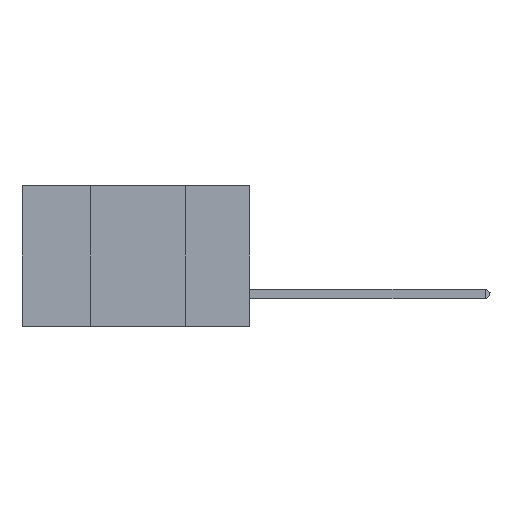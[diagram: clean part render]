
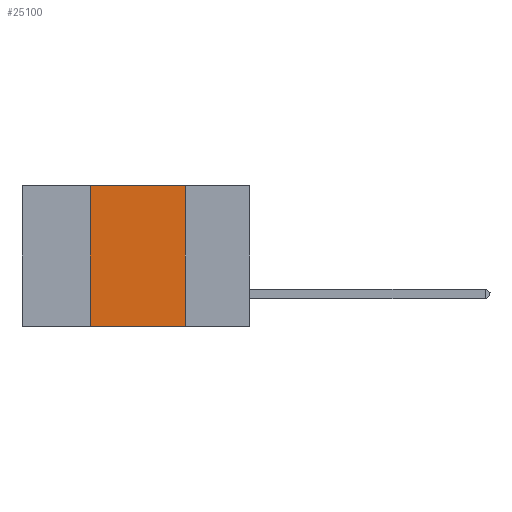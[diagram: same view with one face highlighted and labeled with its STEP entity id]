
A CAD part, left-side view. The second image highlights one B-rep face of the part: STEP entity #25100.
In plain terms, the highlighted planar face has unit normal (-1, 0, 0).
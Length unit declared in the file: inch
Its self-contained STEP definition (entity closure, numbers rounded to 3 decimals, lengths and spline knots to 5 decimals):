
#348 = LINE ( 'NONE', #39843, #4585 ) ;
#433 = VERTEX_POINT ( 'NONE', #11634 ) ;
#893 = DIRECTION ( 'NONE',  ( 0., -1., 0. ) ) ;
#2238 = CARTESIAN_POINT ( 'NONE',  ( 0., 0.42, 0. ) ) ;
#4585 = VECTOR ( 'NONE', #43239, 39.37008 ) ;
#5715 = VECTOR ( 'NONE', #893, 39.37008 ) ;
#5772 = ORIENTED_EDGE ( 'NONE', *, *, #10885, .F. ) ;
#6392 = DIRECTION ( 'NONE',  ( 1., 0., 0. ) ) ;
#7065 = VECTOR ( 'NONE', #43768, 39.37008 ) ;
#7236 = FACE_OUTER_BOUND ( 'NONE', #8734, .T. ) ;
#8734 = EDGE_LOOP ( 'NONE', ( #20968, #5772, #32351, #17614 ) ) ;
#9223 = VERTEX_POINT ( 'NONE', #10938 ) ;
#10885 = EDGE_CURVE ( 'NONE', #35404, #38977, #15616, .T. ) ;
#10938 = CARTESIAN_POINT ( 'NONE',  ( 0., 0.42, -0.37 ) ) ;
#11617 = CARTESIAN_POINT ( 'NONE',  ( 0., 0.6, -0.37 ) ) ;
#11634 = CARTESIAN_POINT ( 'NONE',  ( 0., 0.17, -0.37 ) ) ;
#15448 = CARTESIAN_POINT ( 'NONE',  ( 0., 0.42, 0. ) ) ;
#15616 = LINE ( 'NONE', #40224, #7065 ) ;
#16247 = DIRECTION ( 'NONE',  ( 0., 0., -1. ) ) ;
#17614 = ORIENTED_EDGE ( 'NONE', *, *, #32458, .T. ) ;
#19291 = LINE ( 'NONE', #15448, #34779 ) ;
#20084 = PLANE ( 'NONE',  #43732 ) ;
#20968 = ORIENTED_EDGE ( 'NONE', *, *, #40141, .F. ) ;
#23103 = CARTESIAN_POINT ( 'NONE',  ( 0., 0.17, 0. ) ) ;
#25100 = ADVANCED_FACE ( 'NONE', ( #7236 ), #20084, .F. ) ;
#25852 = DIRECTION ( 'NONE',  ( 0., 0., 1. ) ) ;
#26715 = EDGE_CURVE ( 'NONE', #9223, #35404, #19291, .T. ) ;
#29925 = CARTESIAN_POINT ( 'NONE',  ( 0., 0.6, 0. ) ) ;
#31830 = LINE ( 'NONE', #11617, #5715 ) ;
#32351 = ORIENTED_EDGE ( 'NONE', *, *, #26715, .F. ) ;
#32458 = EDGE_CURVE ( 'NONE', #9223, #433, #31830, .T. ) ;
#34779 = VECTOR ( 'NONE', #25852, 39.37008 ) ;
#35404 = VERTEX_POINT ( 'NONE', #2238 ) ;
#38977 = VERTEX_POINT ( 'NONE', #23103 ) ;
#39843 = CARTESIAN_POINT ( 'NONE',  ( 0., 0.17, 0. ) ) ;
#40141 = EDGE_CURVE ( 'NONE', #38977, #433, #348, .T. ) ;
#40224 = CARTESIAN_POINT ( 'NONE',  ( 0., 0.6, 0. ) ) ;
#43239 = DIRECTION ( 'NONE',  ( 0., 0., -1. ) ) ;
#43732 = AXIS2_PLACEMENT_3D ( 'NONE', #29925, #6392, #16247 ) ;
#43768 = DIRECTION ( 'NONE',  ( 0., -1., 0. ) ) ;
